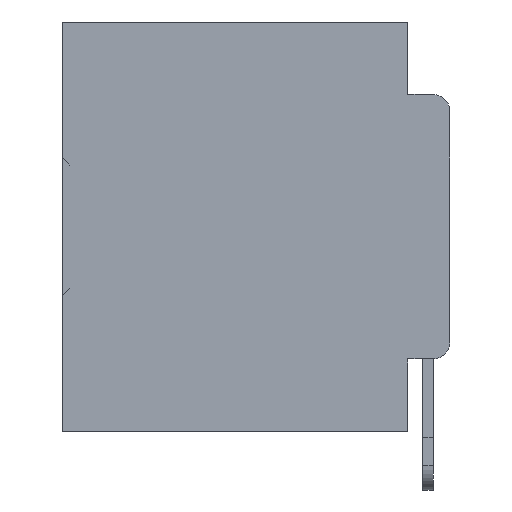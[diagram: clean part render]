
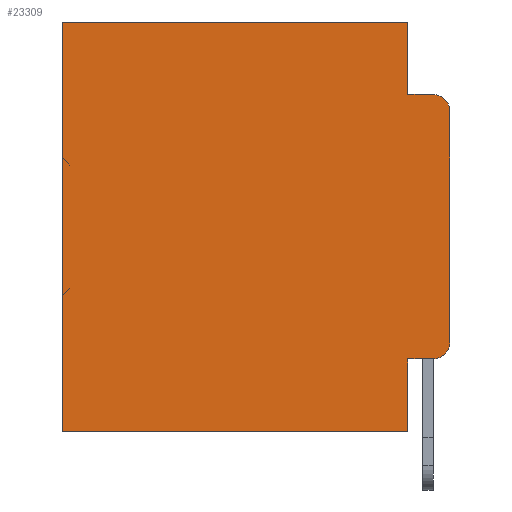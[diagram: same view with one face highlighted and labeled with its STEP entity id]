
A CAD part, left-side view. The second image highlights one B-rep face of the part: STEP entity #23309.
In plain terms, the highlighted planar face has unit normal (-1, 0, 0).
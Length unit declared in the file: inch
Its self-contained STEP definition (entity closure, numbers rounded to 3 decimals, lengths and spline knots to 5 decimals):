
#56 = CARTESIAN_POINT ( 'NONE',  ( 0.298, 0.473, 0. ) ) ;
#302 = VERTEX_POINT ( 'NONE', #3713 ) ;
#904 = CARTESIAN_POINT ( 'NONE',  ( 0.298, 0.02, -0.1085 ) ) ;
#954 = CARTESIAN_POINT ( 'NONE',  ( 0.298, 0., -0.1085 ) ) ;
#1042 = VERTEX_POINT ( 'NONE', #56 ) ;
#1410 = VECTOR ( 'NONE', #19037, 39.37008 ) ;
#1568 = DIRECTION ( 'NONE',  ( 0., 0., -1. ) ) ;
#2405 = VECTOR ( 'NONE', #35476, 39.37008 ) ;
#2713 = ORIENTED_EDGE ( 'NONE', *, *, #16706, .T. ) ;
#3282 = CARTESIAN_POINT ( 'NONE',  ( 0.298, 0.051, 0. ) ) ;
#3713 = CARTESIAN_POINT ( 'NONE',  ( 0.298, 0., -0.3915 ) ) ;
#3736 = FACE_OUTER_BOUND ( 'NONE', #19863, .T. ) ;
#4003 = DIRECTION ( 'NONE',  ( 0., 0., -1. ) ) ;
#4066 = DIRECTION ( 'NONE',  ( 0., -1., 0. ) ) ;
#4358 = LINE ( 'NONE', #26240, #20007 ) ;
#5059 = DIRECTION ( 'NONE',  ( -1., 0., 0. ) ) ;
#5291 = DIRECTION ( 'NONE',  ( 0., 1., 0. ) ) ;
#5353 = DIRECTION ( 'NONE',  ( 0., 0., -1. ) ) ;
#5970 = VECTOR ( 'NONE', #31157, 39.37008 ) ;
#7406 = AXIS2_PLACEMENT_3D ( 'NONE', #22610, #5059, #25499 ) ;
#8053 = EDGE_CURVE ( 'NONE', #14194, #302, #36122, .T. ) ;
#8827 = CIRCLE ( 'NONE', #16848, 0.02 ) ;
#9249 = ORIENTED_EDGE ( 'NONE', *, *, #34054, .F. ) ;
#10427 = LINE ( 'NONE', #32565, #2405 ) ;
#11299 = CARTESIAN_POINT ( 'NONE',  ( 0.298, 0., 0. ) ) ;
#11361 = CARTESIAN_POINT ( 'NONE',  ( 0.298, 0.051, -0.5 ) ) ;
#14186 = CARTESIAN_POINT ( 'NONE',  ( 0.298, 0., 0. ) ) ;
#14194 = VERTEX_POINT ( 'NONE', #954 ) ;
#15747 = VERTEX_POINT ( 'NONE', #3282 ) ;
#16045 = VECTOR ( 'NONE', #4066, 39.37008 ) ;
#16124 = CARTESIAN_POINT ( 'NONE',  ( 0.298, 0.051, 0. ) ) ;
#16706 = EDGE_CURVE ( 'NONE', #30754, #302, #24304, .T. ) ;
#16848 = AXIS2_PLACEMENT_3D ( 'NONE', #904, #21614, #4003 ) ;
#16987 = PLANE ( 'NONE',  #22513 ) ;
#18012 = VERTEX_POINT ( 'NONE', #34623 ) ;
#18302 = VECTOR ( 'NONE', #1568, 39.37008 ) ;
#18639 = EDGE_CURVE ( 'NONE', #25688, #30754, #24602, .T. ) ;
#18794 = CARTESIAN_POINT ( 'NONE',  ( 0.298, 0.051, -0.4115 ) ) ;
#19036 = ORIENTED_EDGE ( 'NONE', *, *, #8053, .F. ) ;
#19037 = DIRECTION ( 'NONE',  ( 0., 0., -1. ) ) ;
#19617 = EDGE_CURVE ( 'NONE', #23321, #18012, #4358, .T. ) ;
#19863 = EDGE_LOOP ( 'NONE', ( #19036, #36635, #23514, #9249, #24057, #24923, #24739, #28900, #31517, #2713 ) ) ;
#20007 = VECTOR ( 'NONE', #37850, 39.37008 ) ;
#20525 = EDGE_CURVE ( 'NONE', #25688, #23321, #24894, .T. ) ;
#21462 = CARTESIAN_POINT ( 'NONE',  ( 0.298, 0.02, -0.0885 ) ) ;
#21614 = DIRECTION ( 'NONE',  ( -1., 0., 0. ) ) ;
#22141 = CARTESIAN_POINT ( 'NONE',  ( 0.298, 0.02, -0.4115 ) ) ;
#22215 = VERTEX_POINT ( 'NONE', #31418 ) ;
#22513 = AXIS2_PLACEMENT_3D ( 'NONE', #14186, #22895, #5353 ) ;
#22610 = CARTESIAN_POINT ( 'NONE',  ( 0.298, 0.02, -0.3915 ) ) ;
#22895 = DIRECTION ( 'NONE',  ( 1., 0., 0. ) ) ;
#23309 = ADVANCED_FACE ( 'NONE', ( #3736 ), #16987, .F. ) ;
#23321 = VERTEX_POINT ( 'NONE', #11361 ) ;
#23514 = ORIENTED_EDGE ( 'NONE', *, *, #36004, .F. ) ;
#24057 = ORIENTED_EDGE ( 'NONE', *, *, #24471, .T. ) ;
#24146 = VERTEX_POINT ( 'NONE', #21462 ) ;
#24304 = CIRCLE ( 'NONE', #7406, 0.02 ) ;
#24414 = EDGE_CURVE ( 'NONE', #1042, #18012, #34190, .T. ) ;
#24471 = EDGE_CURVE ( 'NONE', #15747, #1042, #25624, .T. ) ;
#24602 = LINE ( 'NONE', #18794, #16045 ) ;
#24739 = ORIENTED_EDGE ( 'NONE', *, *, #19617, .F. ) ;
#24894 = LINE ( 'NONE', #16124, #1410 ) ;
#24923 = ORIENTED_EDGE ( 'NONE', *, *, #24414, .T. ) ;
#25104 = CARTESIAN_POINT ( 'NONE',  ( 0.298, 0.051, 0. ) ) ;
#25499 = DIRECTION ( 'NONE',  ( 0., 0., -1. ) ) ;
#25624 = LINE ( 'NONE', #11299, #31495 ) ;
#25688 = VERTEX_POINT ( 'NONE', #31316 ) ;
#26240 = CARTESIAN_POINT ( 'NONE',  ( 0.298, 0., -0.5 ) ) ;
#26854 = DIRECTION ( 'NONE',  ( 0., 0., -1. ) ) ;
#28455 = VECTOR ( 'NONE', #26854, 39.37008 ) ;
#28656 = LINE ( 'NONE', #25104, #18302 ) ;
#28900 = ORIENTED_EDGE ( 'NONE', *, *, #20525, .F. ) ;
#29757 = CARTESIAN_POINT ( 'NONE',  ( 0.298, 0., 0. ) ) ;
#30754 = VERTEX_POINT ( 'NONE', #22141 ) ;
#31157 = DIRECTION ( 'NONE',  ( 0., 0., -1. ) ) ;
#31283 = CARTESIAN_POINT ( 'NONE',  ( 0.298, 0.473, 0. ) ) ;
#31316 = CARTESIAN_POINT ( 'NONE',  ( 0.298, 0.051, -0.4115 ) ) ;
#31418 = CARTESIAN_POINT ( 'NONE',  ( 0.298, 0.051, -0.0885 ) ) ;
#31495 = VECTOR ( 'NONE', #5291, 39.37008 ) ;
#31517 = ORIENTED_EDGE ( 'NONE', *, *, #18639, .T. ) ;
#32565 = CARTESIAN_POINT ( 'NONE',  ( 0.298, 0.051, -0.0885 ) ) ;
#34054 = EDGE_CURVE ( 'NONE', #15747, #22215, #28656, .T. ) ;
#34190 = LINE ( 'NONE', #31283, #5970 ) ;
#34623 = CARTESIAN_POINT ( 'NONE',  ( 0.298, 0.473, -0.5 ) ) ;
#35476 = DIRECTION ( 'NONE',  ( 0., -1., 0. ) ) ;
#36004 = EDGE_CURVE ( 'NONE', #22215, #24146, #10427, .T. ) ;
#36122 = LINE ( 'NONE', #29757, #28455 ) ;
#36635 = ORIENTED_EDGE ( 'NONE', *, *, #37939, .T. ) ;
#37850 = DIRECTION ( 'NONE',  ( 0., 1., 0. ) ) ;
#37939 = EDGE_CURVE ( 'NONE', #14194, #24146, #8827, .T. ) ;
